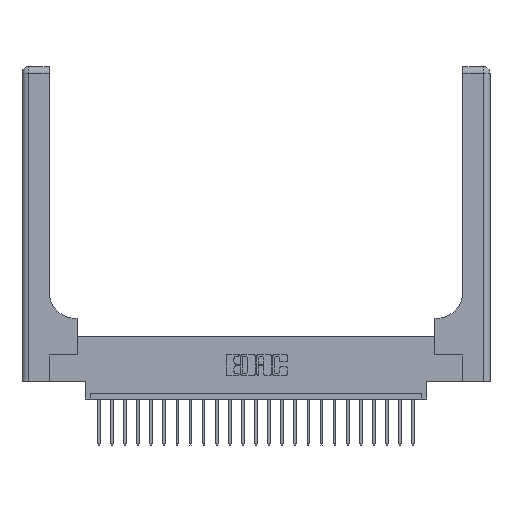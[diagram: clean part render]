
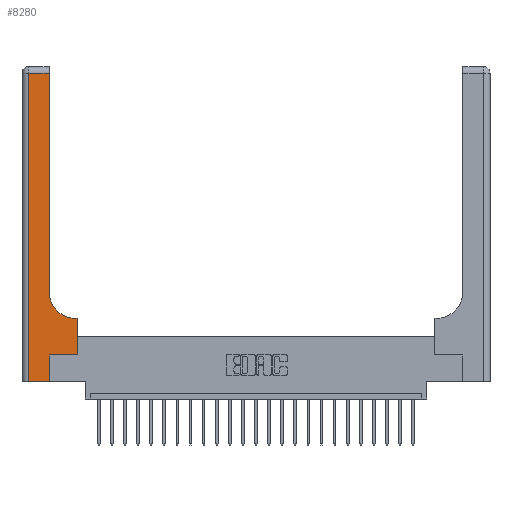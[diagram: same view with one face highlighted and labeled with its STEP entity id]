
A CAD part, top view. The second image highlights one B-rep face of the part: STEP entity #8280.
In plain terms, the highlighted planar face has unit normal (0, 0, 1).
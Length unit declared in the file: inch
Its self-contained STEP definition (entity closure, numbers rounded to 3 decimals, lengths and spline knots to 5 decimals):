
#203 = VECTOR ( 'NONE', #18951, 39.37008 ) ;
#399 = VECTOR ( 'NONE', #692, 39.37008 ) ;
#513 = EDGE_CURVE ( 'NONE', #11759, #16191, #1398, .T. ) ;
#692 = DIRECTION ( 'NONE',  ( 1., 0., 0. ) ) ;
#1018 = VERTEX_POINT ( 'NONE', #22301 ) ;
#1257 = ORIENTED_EDGE ( 'NONE', *, *, #20298, .T. ) ;
#1398 = LINE ( 'NONE', #8122, #17530 ) ;
#1506 = CIRCLE ( 'NONE', #14542, 0.25 ) ;
#1863 = LINE ( 'NONE', #12713, #15838 ) ;
#2005 = DIRECTION ( 'NONE',  ( 1., 0., 0. ) ) ;
#2236 = FACE_OUTER_BOUND ( 'NONE', #14995, .T. ) ;
#2243 = DIRECTION ( 'NONE',  ( 1., 0., 0. ) ) ;
#2887 = CARTESIAN_POINT ( 'NONE',  ( 0.265, 0., 0.37 ) ) ;
#3452 = EDGE_CURVE ( 'NONE', #6754, #17068, #20319, .T. ) ;
#4037 = ORIENTED_EDGE ( 'NONE', *, *, #13333, .T. ) ;
#4651 = CARTESIAN_POINT ( 'NONE',  ( 0.528, 0.25, 0.37 ) ) ;
#5490 = ORIENTED_EDGE ( 'NONE', *, *, #513, .T. ) ;
#5662 = CARTESIAN_POINT ( 'NONE',  ( 0.528, 0.6, 0.37 ) ) ;
#5869 = EDGE_CURVE ( 'NONE', #17323, #1018, #20461, .T. ) ;
#5989 = EDGE_CURVE ( 'NONE', #14801, #16284, #9589, .T. ) ;
#6644 = DIRECTION ( 'NONE',  ( 0., -1., 0. ) ) ;
#6668 = LINE ( 'NONE', #21267, #19500 ) ;
#6754 = VERTEX_POINT ( 'NONE', #11884 ) ;
#8122 = CARTESIAN_POINT ( 'NONE',  ( 0.26, 3., 0.37 ) ) ;
#8280 = ADVANCED_FACE ( 'NONE', ( #2236 ), #12918, .F. ) ;
#8524 = AXIS2_PLACEMENT_3D ( 'NONE', #22371, #21891, #11216 ) ;
#8716 = CARTESIAN_POINT ( 'NONE',  ( 0., 2.94, 0.37 ) ) ;
#9035 = VECTOR ( 'NONE', #9697, 39.37008 ) ;
#9522 = CARTESIAN_POINT ( 'NONE',  ( 0., 0., 0.37 ) ) ;
#9589 = LINE ( 'NONE', #12057, #14062 ) ;
#9697 = DIRECTION ( 'NONE',  ( 0., 1., 0. ) ) ;
#9908 = DIRECTION ( 'NONE',  ( 0., 1., 0. ) ) ;
#10374 = CARTESIAN_POINT ( 'NONE',  ( 0.06, 2.94, 0.37 ) ) ;
#10831 = CARTESIAN_POINT ( 'NONE',  ( 0.51, 0.6, 0.37 ) ) ;
#11216 = DIRECTION ( 'NONE',  ( -1., 0., 0. ) ) ;
#11299 = DIRECTION ( 'NONE',  ( 0., 0., -1. ) ) ;
#11659 = CARTESIAN_POINT ( 'NONE',  ( 0.265, 0., 0.37 ) ) ;
#11759 = VERTEX_POINT ( 'NONE', #19031 ) ;
#11884 = CARTESIAN_POINT ( 'NONE',  ( 0.528, 0.25, 0.37 ) ) ;
#12057 = CARTESIAN_POINT ( 'NONE',  ( 0.06, 3., 0.37 ) ) ;
#12239 = DIRECTION ( 'NONE',  ( -1., 0., 0. ) ) ;
#12713 = CARTESIAN_POINT ( 'NONE',  ( 0.265, 0.25, 0.37 ) ) ;
#12918 = PLANE ( 'NONE',  #8524 ) ;
#13333 = EDGE_CURVE ( 'NONE', #16191, #14801, #22692, .T. ) ;
#13505 = CARTESIAN_POINT ( 'NONE',  ( 0.26, 2.94, 0.37 ) ) ;
#13538 = LINE ( 'NONE', #9522, #399 ) ;
#13820 = EDGE_CURVE ( 'NONE', #17068, #17524, #6668, .T. ) ;
#14062 = VECTOR ( 'NONE', #6644, 39.37008 ) ;
#14542 = AXIS2_PLACEMENT_3D ( 'NONE', #14875, #11299, #2243 ) ;
#14801 = VERTEX_POINT ( 'NONE', #10374 ) ;
#14875 = CARTESIAN_POINT ( 'NONE',  ( 0.51, 0.85, 0.37 ) ) ;
#14995 = EDGE_LOOP ( 'NONE', ( #5490, #4037, #22368, #17555, #22203, #21985, #20436, #17252, #1257 ) ) ;
#15838 = VECTOR ( 'NONE', #2005, 39.37008 ) ;
#16158 = EDGE_CURVE ( 'NONE', #16284, #17323, #13538, .T. ) ;
#16191 = VERTEX_POINT ( 'NONE', #13505 ) ;
#16284 = VERTEX_POINT ( 'NONE', #20673 ) ;
#16795 = VECTOR ( 'NONE', #12239, 39.37008 ) ;
#17068 = VERTEX_POINT ( 'NONE', #5662 ) ;
#17252 = ORIENTED_EDGE ( 'NONE', *, *, #13820, .T. ) ;
#17323 = VERTEX_POINT ( 'NONE', #2887 ) ;
#17524 = VERTEX_POINT ( 'NONE', #10831 ) ;
#17530 = VECTOR ( 'NONE', #9908, 39.37008 ) ;
#17555 = ORIENTED_EDGE ( 'NONE', *, *, #16158, .T. ) ;
#18951 = DIRECTION ( 'NONE',  ( 0., 1., 0. ) ) ;
#19031 = CARTESIAN_POINT ( 'NONE',  ( 0.26, 0.85, 0.37 ) ) ;
#19381 = DIRECTION ( 'NONE',  ( -1., 0., 0. ) ) ;
#19500 = VECTOR ( 'NONE', #19381, 39.37008 ) ;
#20117 = EDGE_CURVE ( 'NONE', #1018, #6754, #1863, .T. ) ;
#20298 = EDGE_CURVE ( 'NONE', #17524, #11759, #1506, .T. ) ;
#20319 = LINE ( 'NONE', #4651, #203 ) ;
#20436 = ORIENTED_EDGE ( 'NONE', *, *, #3452, .T. ) ;
#20461 = LINE ( 'NONE', #11659, #9035 ) ;
#20673 = CARTESIAN_POINT ( 'NONE',  ( 0.06, 0., 0.37 ) ) ;
#21267 = CARTESIAN_POINT ( 'NONE',  ( 0.26, 0.6, 0.37 ) ) ;
#21891 = DIRECTION ( 'NONE',  ( 0., 0., -1. ) ) ;
#21985 = ORIENTED_EDGE ( 'NONE', *, *, #20117, .T. ) ;
#22203 = ORIENTED_EDGE ( 'NONE', *, *, #5869, .T. ) ;
#22301 = CARTESIAN_POINT ( 'NONE',  ( 0.265, 0.25, 0.37 ) ) ;
#22368 = ORIENTED_EDGE ( 'NONE', *, *, #5989, .T. ) ;
#22371 = CARTESIAN_POINT ( 'NONE',  ( 0., 3., 0.37 ) ) ;
#22692 = LINE ( 'NONE', #8716, #16795 ) ;
